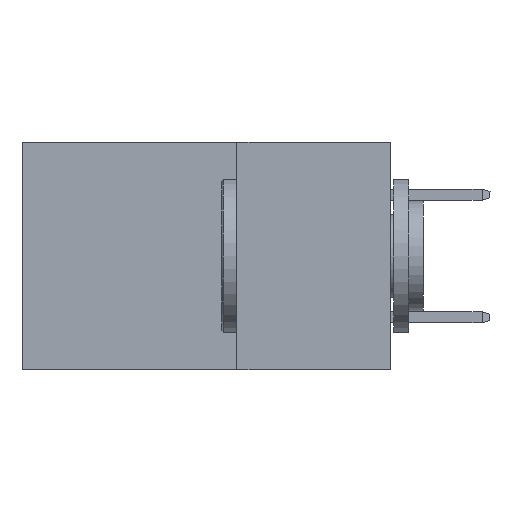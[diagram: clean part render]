
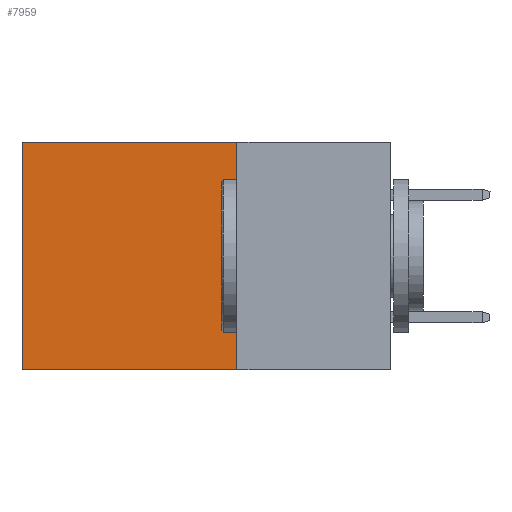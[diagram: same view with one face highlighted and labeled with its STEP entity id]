
A CAD part, left-side view. The second image highlights one B-rep face of the part: STEP entity #7959.
In plain terms, the highlighted planar face has unit normal (-1, 0, 0).
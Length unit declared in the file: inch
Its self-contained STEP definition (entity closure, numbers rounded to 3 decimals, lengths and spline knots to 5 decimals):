
#216 = CARTESIAN_POINT ( 'NONE',  ( 0.2875, 0.25, 0. ) ) ;
#953 = EDGE_CURVE ( 'NONE', #15899, #3976, #7892, .T. ) ;
#1513 = DIRECTION ( 'NONE',  ( 0., 0., -1. ) ) ;
#2217 = VECTOR ( 'NONE', #15428, 39.37008 ) ;
#2696 = CARTESIAN_POINT ( 'NONE',  ( 0.2875, 0.6, -0.37 ) ) ;
#3572 = LINE ( 'NONE', #3772, #12716 ) ;
#3772 = CARTESIAN_POINT ( 'NONE',  ( 0.2875, 0.6, 0. ) ) ;
#3976 = VERTEX_POINT ( 'NONE', #6445 ) ;
#4124 = VERTEX_POINT ( 'NONE', #11675 ) ;
#4526 = CARTESIAN_POINT ( 'NONE',  ( 0.2875, 0.25, 0. ) ) ;
#4943 = VECTOR ( 'NONE', #8523, 39.37008 ) ;
#5150 = ORIENTED_EDGE ( 'NONE', *, *, #7299, .T. ) ;
#5271 = VECTOR ( 'NONE', #9874, 39.37008 ) ;
#6335 = VERTEX_POINT ( 'NONE', #2696 ) ;
#6388 = ORIENTED_EDGE ( 'NONE', *, *, #10558, .T. ) ;
#6445 = CARTESIAN_POINT ( 'NONE',  ( 0.2875, 0.25, -0.37 ) ) ;
#7265 = CARTESIAN_POINT ( 'NONE',  ( 0.2875, 0.25, -0.37 ) ) ;
#7299 = EDGE_CURVE ( 'NONE', #4124, #6335, #3572, .T. ) ;
#7892 = LINE ( 'NONE', #9064, #5271 ) ;
#7959 = ADVANCED_FACE ( 'NONE', ( #15008 ), #12706, .F. ) ;
#8523 = DIRECTION ( 'NONE',  ( 0., 1., 0. ) ) ;
#9064 = CARTESIAN_POINT ( 'NONE',  ( 0.2875, 0.25, 0. ) ) ;
#9166 = DIRECTION ( 'NONE',  ( 1., 0., 0. ) ) ;
#9874 = DIRECTION ( 'NONE',  ( 0., 0., -1. ) ) ;
#10558 = EDGE_CURVE ( 'NONE', #15899, #4124, #12177, .T. ) ;
#11265 = DIRECTION ( 'NONE',  ( 0., 0., -1. ) ) ;
#11675 = CARTESIAN_POINT ( 'NONE',  ( 0.2875, 0.6, 0. ) ) ;
#12073 = AXIS2_PLACEMENT_3D ( 'NONE', #216, #9166, #1513 ) ;
#12177 = LINE ( 'NONE', #12950, #2217 ) ;
#12477 = ORIENTED_EDGE ( 'NONE', *, *, #953, .F. ) ;
#12658 = EDGE_LOOP ( 'NONE', ( #5150, #15001, #12477, #6388 ) ) ;
#12706 = PLANE ( 'NONE',  #12073 ) ;
#12716 = VECTOR ( 'NONE', #11265, 39.37008 ) ;
#12826 = EDGE_CURVE ( 'NONE', #3976, #6335, #14417, .T. ) ;
#12950 = CARTESIAN_POINT ( 'NONE',  ( 0.2875, 0.25, 0. ) ) ;
#14417 = LINE ( 'NONE', #7265, #4943 ) ;
#15001 = ORIENTED_EDGE ( 'NONE', *, *, #12826, .F. ) ;
#15008 = FACE_OUTER_BOUND ( 'NONE', #12658, .T. ) ;
#15428 = DIRECTION ( 'NONE',  ( 0., 1., 0. ) ) ;
#15899 = VERTEX_POINT ( 'NONE', #4526 ) ;
